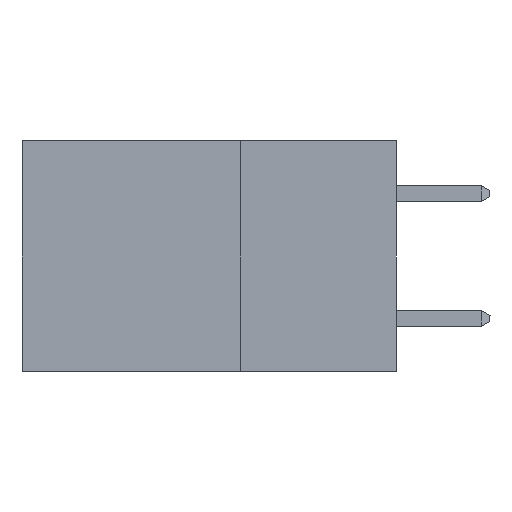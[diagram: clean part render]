
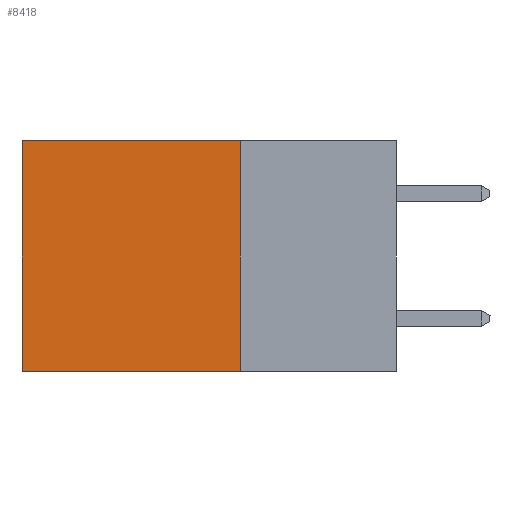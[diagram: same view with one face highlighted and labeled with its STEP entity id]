
A CAD part, left-side view. The second image highlights one B-rep face of the part: STEP entity #8418.
In plain terms, the highlighted planar face has unit normal (-1, 0, 0).
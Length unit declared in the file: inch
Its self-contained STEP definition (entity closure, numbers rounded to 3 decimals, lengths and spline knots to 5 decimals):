
#294 = FACE_OUTER_BOUND ( 'NONE', #5157, .T. ) ;
#579 = EDGE_CURVE ( 'NONE', #6746, #2888, #11345, .T. ) ;
#956 = DIRECTION ( 'NONE',  ( 0., 0., -1. ) ) ;
#1658 = ORIENTED_EDGE ( 'NONE', *, *, #11635, .F. ) ;
#1686 = VERTEX_POINT ( 'NONE', #13079 ) ;
#1761 = LINE ( 'NONE', #7004, #2406 ) ;
#1776 = LINE ( 'NONE', #2488, #6986 ) ;
#2058 = ORIENTED_EDGE ( 'NONE', *, *, #4511, .F. ) ;
#2406 = VECTOR ( 'NONE', #6987, 39.37008 ) ;
#2488 = CARTESIAN_POINT ( 'NONE',  ( 0.2615, 0.25, -0.37 ) ) ;
#2888 = VERTEX_POINT ( 'NONE', #11145 ) ;
#3129 = VECTOR ( 'NONE', #956, 39.37008 ) ;
#4412 = DIRECTION ( 'NONE',  ( 0., 0., -1. ) ) ;
#4511 = EDGE_CURVE ( 'NONE', #1686, #5853, #1776, .T. ) ;
#4514 = AXIS2_PLACEMENT_3D ( 'NONE', #10656, #10156, #10138 ) ;
#4755 = ORIENTED_EDGE ( 'NONE', *, *, #579, .T. ) ;
#4931 = EDGE_CURVE ( 'NONE', #1686, #6746, #1761, .T. ) ;
#5157 = EDGE_LOOP ( 'NONE', ( #4755, #1658, #2058, #9904 ) ) ;
#5853 = VERTEX_POINT ( 'NONE', #7182 ) ;
#6393 = DIRECTION ( 'NONE',  ( 0., 1., 0. ) ) ;
#6619 = CARTESIAN_POINT ( 'NONE',  ( 0.2615, 0.25, -0.37 ) ) ;
#6746 = VERTEX_POINT ( 'NONE', #6912 ) ;
#6912 = CARTESIAN_POINT ( 'NONE',  ( 0.2615, 0.6, 0. ) ) ;
#6986 = VECTOR ( 'NONE', #4412, 39.37008 ) ;
#6987 = DIRECTION ( 'NONE',  ( 0., 1., 0. ) ) ;
#7004 = CARTESIAN_POINT ( 'NONE',  ( 0.2615, 0.25, 0. ) ) ;
#7182 = CARTESIAN_POINT ( 'NONE',  ( 0.2615, 0.25, -0.37 ) ) ;
#8329 = CARTESIAN_POINT ( 'NONE',  ( 0.2615, 0.6, -0.37 ) ) ;
#8418 = ADVANCED_FACE ( 'NONE', ( #294 ), #10194, .F. ) ;
#9557 = LINE ( 'NONE', #6619, #11759 ) ;
#9904 = ORIENTED_EDGE ( 'NONE', *, *, #4931, .T. ) ;
#10138 = DIRECTION ( 'NONE',  ( 0., 0., -1. ) ) ;
#10156 = DIRECTION ( 'NONE',  ( 1., 0., 0. ) ) ;
#10194 = PLANE ( 'NONE',  #4514 ) ;
#10656 = CARTESIAN_POINT ( 'NONE',  ( 0.2615, 0.25, -0.37 ) ) ;
#11145 = CARTESIAN_POINT ( 'NONE',  ( 0.2615, 0.6, -0.37 ) ) ;
#11345 = LINE ( 'NONE', #8329, #3129 ) ;
#11635 = EDGE_CURVE ( 'NONE', #5853, #2888, #9557, .T. ) ;
#11759 = VECTOR ( 'NONE', #6393, 39.37008 ) ;
#13079 = CARTESIAN_POINT ( 'NONE',  ( 0.2615, 0.25, 0. ) ) ;
